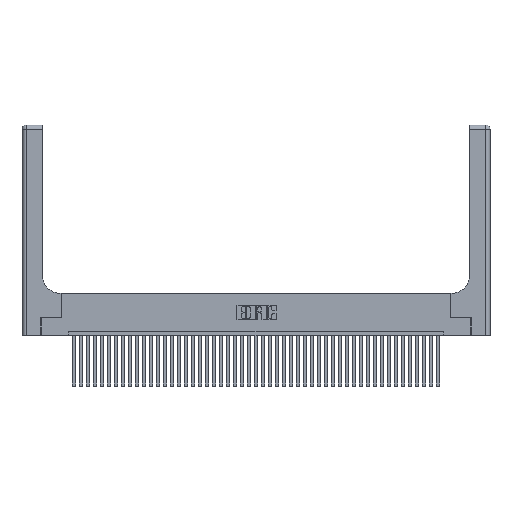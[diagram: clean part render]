
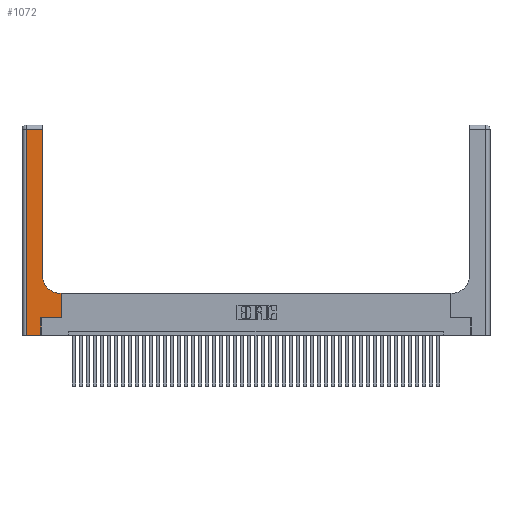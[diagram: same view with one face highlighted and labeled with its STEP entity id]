
A CAD part, top view. The second image highlights one B-rep face of the part: STEP entity #1072.
In plain terms, the highlighted planar face has unit normal (0, 0, 1).
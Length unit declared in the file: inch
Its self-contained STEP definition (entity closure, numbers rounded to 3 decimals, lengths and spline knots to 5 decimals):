
#1072 = ADVANCED_FACE ( 'NONE', ( #5991 ), #2552, .F. ) ;
#2552 = PLANE ( 'NONE',  #20928 ) ;
#2726 = DIRECTION ( 'NONE',  ( -1., 0., 0. ) ) ;
#2729 = VECTOR ( 'NONE', #32516, 39.37008 ) ;
#2816 = VECTOR ( 'NONE', #34125, 39.37008 ) ;
#2832 = EDGE_CURVE ( 'NONE', #27962, #18186, #39566, .T. ) ;
#3762 = EDGE_LOOP ( 'NONE', ( #17055, #39236, #36918, #38263, #7414, #25563, #14865, #13105, #33086 ) ) ;
#3930 = EDGE_CURVE ( 'NONE', #41611, #37404, #8008, .T. ) ;
#5910 = CARTESIAN_POINT ( 'NONE',  ( 0.5585, 0.25, 0.37 ) ) ;
#5936 = CARTESIAN_POINT ( 'NONE',  ( 0., 3., 0.37 ) ) ;
#5991 = FACE_OUTER_BOUND ( 'NONE', #3762, .T. ) ;
#6298 = CARTESIAN_POINT ( 'NONE',  ( 0.2915, 0.6, 0.37 ) ) ;
#7140 = VERTEX_POINT ( 'NONE', #37170 ) ;
#7414 = ORIENTED_EDGE ( 'NONE', *, *, #3930, .T. ) ;
#7590 = EDGE_CURVE ( 'NONE', #37404, #31879, #25222, .T. ) ;
#8008 = LINE ( 'NONE', #37193, #2816 ) ;
#8732 = EDGE_CURVE ( 'NONE', #18186, #23399, #40063, .T. ) ;
#9282 = DIRECTION ( 'NONE',  ( 0., 0., -1. ) ) ;
#9910 = DIRECTION ( 'NONE',  ( 0., 0., -1. ) ) ;
#10918 = DIRECTION ( 'NONE',  ( 0., -1., 0. ) ) ;
#11448 = CARTESIAN_POINT ( 'NONE',  ( 0.269, 0., 0.37 ) ) ;
#12698 = DIRECTION ( 'NONE',  ( -1., 0., 0. ) ) ;
#13105 = ORIENTED_EDGE ( 'NONE', *, *, #27581, .T. ) ;
#13534 = LINE ( 'NONE', #14682, #23904 ) ;
#13906 = AXIS2_PLACEMENT_3D ( 'NONE', #36771, #9910, #30180 ) ;
#13911 = VECTOR ( 'NONE', #2726, 39.37008 ) ;
#14462 = EDGE_CURVE ( 'NONE', #23643, #27962, #16213, .T. ) ;
#14682 = CARTESIAN_POINT ( 'NONE',  ( 0., 0., 0.37 ) ) ;
#14865 = ORIENTED_EDGE ( 'NONE', *, *, #19072, .T. ) ;
#15203 = LINE ( 'NONE', #5910, #22001 ) ;
#16213 = LINE ( 'NONE', #20371, #33964 ) ;
#17055 = ORIENTED_EDGE ( 'NONE', *, *, #14462, .T. ) ;
#18186 = VERTEX_POINT ( 'NONE', #34383 ) ;
#18490 = CARTESIAN_POINT ( 'NONE',  ( 0.269, 0.25, 0.37 ) ) ;
#19072 = EDGE_CURVE ( 'NONE', #31879, #7140, #15203, .T. ) ;
#20371 = CARTESIAN_POINT ( 'NONE',  ( 0.2915, 3., 0.37 ) ) ;
#20928 = AXIS2_PLACEMENT_3D ( 'NONE', #5936, #9282, #35447 ) ;
#22001 = VECTOR ( 'NONE', #29386, 39.37008 ) ;
#22266 = CARTESIAN_POINT ( 'NONE',  ( 0.269, 0.25, 0.37 ) ) ;
#23399 = VERTEX_POINT ( 'NONE', #32752 ) ;
#23643 = VERTEX_POINT ( 'NONE', #39289 ) ;
#23904 = VECTOR ( 'NONE', #38074, 39.37008 ) ;
#24599 = CARTESIAN_POINT ( 'NONE',  ( 0.2915, 2.94, 0.37 ) ) ;
#25019 = VECTOR ( 'NONE', #12698, 39.37008 ) ;
#25222 = LINE ( 'NONE', #22266, #2729 ) ;
#25563 = ORIENTED_EDGE ( 'NONE', *, *, #7590, .T. ) ;
#27581 = EDGE_CURVE ( 'NONE', #7140, #31268, #29222, .T. ) ;
#27952 = EDGE_CURVE ( 'NONE', #23399, #41611, #13534, .T. ) ;
#27962 = VERTEX_POINT ( 'NONE', #24599 ) ;
#28502 = VECTOR ( 'NONE', #10918, 39.37008 ) ;
#29222 = LINE ( 'NONE', #6298, #25019 ) ;
#29386 = DIRECTION ( 'NONE',  ( 0., 1., 0. ) ) ;
#29873 = DIRECTION ( 'NONE',  ( 0., 1., 0. ) ) ;
#30180 = DIRECTION ( 'NONE',  ( 1., 0., 0. ) ) ;
#31268 = VERTEX_POINT ( 'NONE', #36328 ) ;
#31879 = VERTEX_POINT ( 'NONE', #43038 ) ;
#32250 = CARTESIAN_POINT ( 'NONE',  ( 0., 2.94, 0.37 ) ) ;
#32516 = DIRECTION ( 'NONE',  ( 1., 0., 0. ) ) ;
#32752 = CARTESIAN_POINT ( 'NONE',  ( 0.06, 0., 0.37 ) ) ;
#33086 = ORIENTED_EDGE ( 'NONE', *, *, #38765, .T. ) ;
#33964 = VECTOR ( 'NONE', #29873, 39.37008 ) ;
#34125 = DIRECTION ( 'NONE',  ( 0., 1., 0. ) ) ;
#34161 = CARTESIAN_POINT ( 'NONE',  ( 0.06, 3., 0.37 ) ) ;
#34383 = CARTESIAN_POINT ( 'NONE',  ( 0.06, 2.94, 0.37 ) ) ;
#35447 = DIRECTION ( 'NONE',  ( -1., 0., 0. ) ) ;
#35553 = CIRCLE ( 'NONE', #13906, 0.25 ) ;
#36328 = CARTESIAN_POINT ( 'NONE',  ( 0.5415, 0.6, 0.37 ) ) ;
#36771 = CARTESIAN_POINT ( 'NONE',  ( 0.5415, 0.85, 0.37 ) ) ;
#36918 = ORIENTED_EDGE ( 'NONE', *, *, #8732, .T. ) ;
#37170 = CARTESIAN_POINT ( 'NONE',  ( 0.5585, 0.6, 0.37 ) ) ;
#37193 = CARTESIAN_POINT ( 'NONE',  ( 0.269, 0., 0.37 ) ) ;
#37404 = VERTEX_POINT ( 'NONE', #18490 ) ;
#38074 = DIRECTION ( 'NONE',  ( 1., 0., 0. ) ) ;
#38263 = ORIENTED_EDGE ( 'NONE', *, *, #27952, .T. ) ;
#38765 = EDGE_CURVE ( 'NONE', #31268, #23643, #35553, .T. ) ;
#39236 = ORIENTED_EDGE ( 'NONE', *, *, #2832, .T. ) ;
#39289 = CARTESIAN_POINT ( 'NONE',  ( 0.2915, 0.85, 0.37 ) ) ;
#39566 = LINE ( 'NONE', #32250, #13911 ) ;
#40063 = LINE ( 'NONE', #34161, #28502 ) ;
#41611 = VERTEX_POINT ( 'NONE', #11448 ) ;
#43038 = CARTESIAN_POINT ( 'NONE',  ( 0.5585, 0.25, 0.37 ) ) ;
